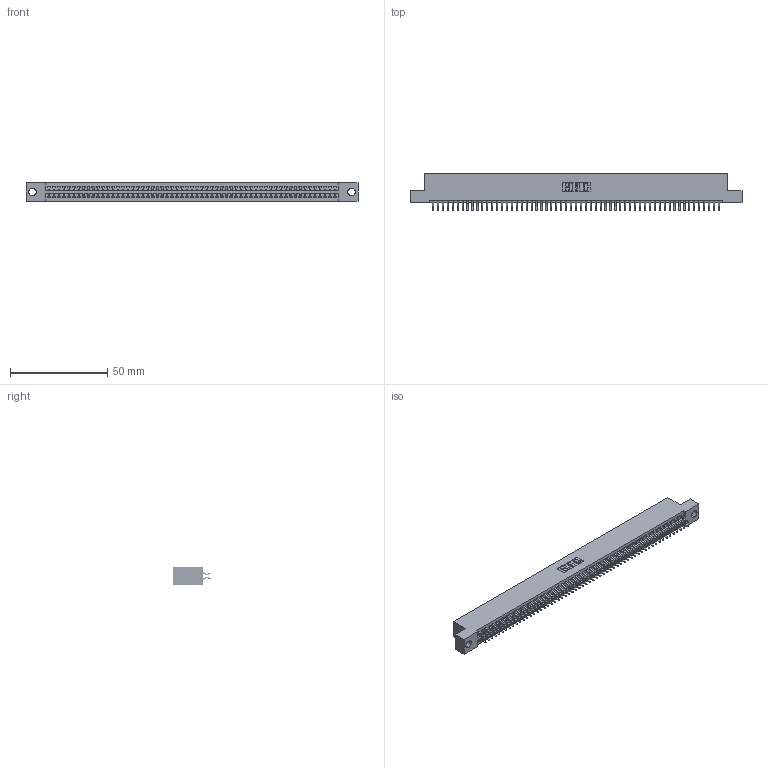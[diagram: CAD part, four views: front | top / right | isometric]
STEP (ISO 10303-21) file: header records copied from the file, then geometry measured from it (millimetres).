
FILE_DESCRIPTION (( 'STEP AP203' ), '1' );
FILE_NAME ('345-118-556-204.STEP', '2021-05-25T16:28:56', ( '' ), ( '' ), 'SwSTEP 2.0', 'SolidWorks 2020', '' );
FILE_SCHEMA (( 'CONFIG_CONTROL_DESIGN' ));
Length unit declared in the file: inch
Products named in the file (3): 345-118-556-204; 345-292-001_556 Tail; 345 Part_Flush Mounting Lugs - 0.156 Dia-TI
Assembly tree (119 placements, depth 2):
  345-118-556-204
    345 Part_Flush Mounting Lugs - 0.156 Dia-TI
    345-292-001_556 Tail  x118
Bounding box: 171.07 x 19.24 x 9.4 mm (x, y, z)
Volume: 16665 mm3; surface area: 24711.2 mm2
Topology: 119 solids, 119 shells, 6748 faces, 20083 edges, 13230 vertices
Faces by surface type: plane 4460, cylinder 2288
Entity records: 44643 total; most frequent: CARTESIAN_POINT 7486, ORIENTED_EDGE 7406, DIRECTION 6567, EDGE_CURVE 3703, VECTOR 3327, LINE 3327, VERTEX_POINT 2466, AXIS2_PLACEMENT_3D 1620
